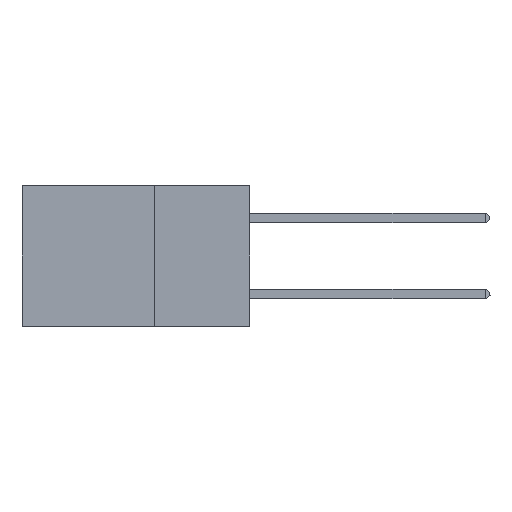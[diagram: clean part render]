
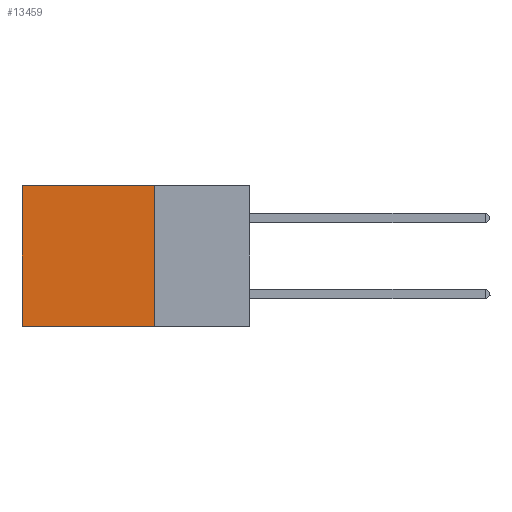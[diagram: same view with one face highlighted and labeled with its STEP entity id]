
A CAD part, left-side view. The second image highlights one B-rep face of the part: STEP entity #13459.
In plain terms, the highlighted planar face has unit normal (-1, 0, 0).
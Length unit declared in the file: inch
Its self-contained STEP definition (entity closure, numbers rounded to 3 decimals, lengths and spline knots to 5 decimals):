
#110 = VERTEX_POINT ( 'NONE', #5220 ) ;
#559 = CARTESIAN_POINT ( 'NONE',  ( 0.2875, 0.25, 0. ) ) ;
#1187 = VERTEX_POINT ( 'NONE', #30537 ) ;
#1693 = ORIENTED_EDGE ( 'NONE', *, *, #3129, .T. ) ;
#2844 = FACE_OUTER_BOUND ( 'NONE', #34593, .T. ) ;
#2885 = VECTOR ( 'NONE', #14794, 39.37008 ) ;
#3129 = EDGE_CURVE ( 'NONE', #110, #10374, #4122, .T. ) ;
#4122 = LINE ( 'NONE', #19034, #12068 ) ;
#5220 = CARTESIAN_POINT ( 'NONE',  ( 0.2875, 0.6, 0. ) ) ;
#8515 = EDGE_CURVE ( 'NONE', #34892, #10374, #18861, .T. ) ;
#8576 = CARTESIAN_POINT ( 'NONE',  ( 0.2875, 0.25, 0. ) ) ;
#9250 = VECTOR ( 'NONE', #33620, 39.37008 ) ;
#10374 = VERTEX_POINT ( 'NONE', #11432 ) ;
#11223 = LINE ( 'NONE', #8576, #2885 ) ;
#11432 = CARTESIAN_POINT ( 'NONE',  ( 0.2875, 0.6, -0.37 ) ) ;
#12001 = EDGE_CURVE ( 'NONE', #1187, #110, #27788, .T. ) ;
#12068 = VECTOR ( 'NONE', #15796, 39.37008 ) ;
#13459 = ADVANCED_FACE ( 'NONE', ( #2844 ), #32096, .F. ) ;
#14794 = DIRECTION ( 'NONE',  ( 0., 0., -1. ) ) ;
#15552 = VECTOR ( 'NONE', #36592, 39.37008 ) ;
#15796 = DIRECTION ( 'NONE',  ( 0., 0., -1. ) ) ;
#16614 = CARTESIAN_POINT ( 'NONE',  ( 0.2875, 0.25, 0. ) ) ;
#18861 = LINE ( 'NONE', #30375, #15552 ) ;
#19034 = CARTESIAN_POINT ( 'NONE',  ( 0.2875, 0.6, 0. ) ) ;
#19795 = CARTESIAN_POINT ( 'NONE',  ( 0.2875, 0.25, -0.37 ) ) ;
#26278 = DIRECTION ( 'NONE',  ( 1., 0., 0. ) ) ;
#27788 = LINE ( 'NONE', #16614, #9250 ) ;
#27827 = AXIS2_PLACEMENT_3D ( 'NONE', #559, #26278, #29087 ) ;
#29087 = DIRECTION ( 'NONE',  ( 0., 0., -1. ) ) ;
#30375 = CARTESIAN_POINT ( 'NONE',  ( 0.2875, 0.25, -0.37 ) ) ;
#30537 = CARTESIAN_POINT ( 'NONE',  ( 0.2875, 0.25, 0. ) ) ;
#31064 = ORIENTED_EDGE ( 'NONE', *, *, #8515, .F. ) ;
#31483 = ORIENTED_EDGE ( 'NONE', *, *, #35369, .F. ) ;
#32096 = PLANE ( 'NONE',  #27827 ) ;
#33620 = DIRECTION ( 'NONE',  ( 0., 1., 0. ) ) ;
#34448 = ORIENTED_EDGE ( 'NONE', *, *, #12001, .T. ) ;
#34593 = EDGE_LOOP ( 'NONE', ( #1693, #31064, #31483, #34448 ) ) ;
#34892 = VERTEX_POINT ( 'NONE', #19795 ) ;
#35369 = EDGE_CURVE ( 'NONE', #1187, #34892, #11223, .T. ) ;
#36592 = DIRECTION ( 'NONE',  ( 0., 1., 0. ) ) ;
